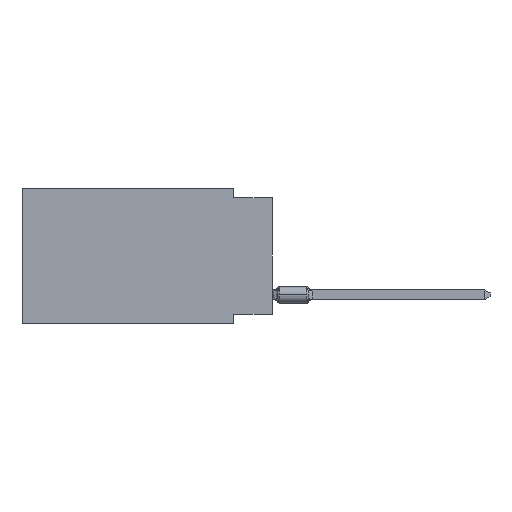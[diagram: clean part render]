
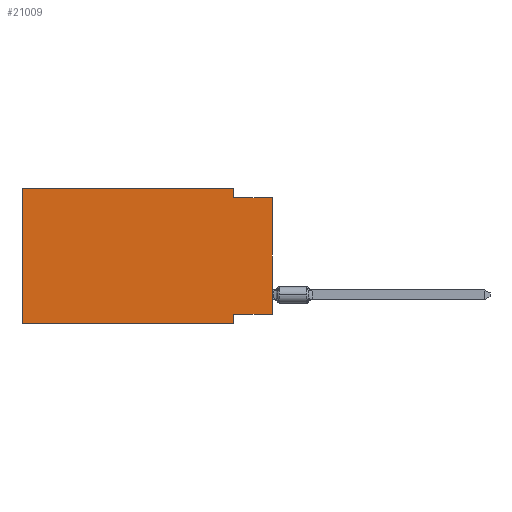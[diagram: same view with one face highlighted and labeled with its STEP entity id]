
A CAD part, left-side view. The second image highlights one B-rep face of the part: STEP entity #21009.
In plain terms, the highlighted planar face has unit normal (-1, 0, 0).
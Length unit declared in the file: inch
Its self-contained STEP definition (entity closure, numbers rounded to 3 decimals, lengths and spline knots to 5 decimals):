
#61 = CARTESIAN_POINT ( 'NONE',  ( 0., 0.645, 0. ) ) ;
#374 = EDGE_CURVE ( 'NONE', #6343, #25989, #20993, .T. ) ;
#680 = ORIENTED_EDGE ( 'NONE', *, *, #27275, .F. ) ;
#3112 = VECTOR ( 'NONE', #25550, 39.37008 ) ;
#3421 = DIRECTION ( 'NONE',  ( 1., 0., 0. ) ) ;
#3566 = CARTESIAN_POINT ( 'NONE',  ( 0., 0.645, 0. ) ) ;
#4497 = EDGE_CURVE ( 'NONE', #8063, #25989, #25173, .T. ) ;
#6343 = VERTEX_POINT ( 'NONE', #27596 ) ;
#6353 = VERTEX_POINT ( 'NONE', #24683 ) ;
#8007 = EDGE_CURVE ( 'NONE', #20018, #30855, #15881, .T. ) ;
#8063 = VERTEX_POINT ( 'NONE', #21209 ) ;
#8248 = VECTOR ( 'NONE', #24848, 39.37008 ) ;
#9344 = ORIENTED_EDGE ( 'NONE', *, *, #4497, .T. ) ;
#10070 = EDGE_CURVE ( 'NONE', #20807, #30855, #14075, .T. ) ;
#10418 = CARTESIAN_POINT ( 'NONE',  ( 0., 0.645, -0.35 ) ) ;
#10787 = AXIS2_PLACEMENT_3D ( 'NONE', #3566, #3421, #30625 ) ;
#10837 = ORIENTED_EDGE ( 'NONE', *, *, #8007, .T. ) ;
#11301 = DIRECTION ( 'NONE',  ( 0., -1., 0. ) ) ;
#12290 = CARTESIAN_POINT ( 'NONE',  ( 0., 0., -0.025 ) ) ;
#13291 = DIRECTION ( 'NONE',  ( 0., 0., 1. ) ) ;
#13655 = VECTOR ( 'NONE', #13291, 39.37008 ) ;
#14075 = LINE ( 'NONE', #19092, #23064 ) ;
#14401 = ORIENTED_EDGE ( 'NONE', *, *, #29085, .F. ) ;
#14994 = DIRECTION ( 'NONE',  ( 0., -1., 0. ) ) ;
#15822 = CARTESIAN_POINT ( 'NONE',  ( 0., 0.1, -0.35 ) ) ;
#15881 = LINE ( 'NONE', #20422, #13655 ) ;
#17553 = ORIENTED_EDGE ( 'NONE', *, *, #25008, .F. ) ;
#18621 = FACE_OUTER_BOUND ( 'NONE', #28024, .T. ) ;
#19092 = CARTESIAN_POINT ( 'NONE',  ( 0., 0., -0.025 ) ) ;
#19702 = DIRECTION ( 'NONE',  ( 0., 0., -1. ) ) ;
#19790 = CARTESIAN_POINT ( 'NONE',  ( 0., 0.1, -0.025 ) ) ;
#20018 = VERTEX_POINT ( 'NONE', #24718 ) ;
#20422 = CARTESIAN_POINT ( 'NONE',  ( 0., 0., 0. ) ) ;
#20581 = CARTESIAN_POINT ( 'NONE',  ( 0., 0.645, 0. ) ) ;
#20807 = VERTEX_POINT ( 'NONE', #19790 ) ;
#20993 = LINE ( 'NONE', #15822, #3112 ) ;
#21009 = ADVANCED_FACE ( 'NONE', ( #18621 ), #30462, .F. ) ;
#21209 = CARTESIAN_POINT ( 'NONE',  ( 0., 0.645, -0.35 ) ) ;
#21732 = CARTESIAN_POINT ( 'NONE',  ( 0., 0.1, -0.35 ) ) ;
#21948 = VECTOR ( 'NONE', #23014, 39.37008 ) ;
#22127 = CARTESIAN_POINT ( 'NONE',  ( 0., 0.645, 0. ) ) ;
#23014 = DIRECTION ( 'NONE',  ( 0., 0., 1. ) ) ;
#23064 = VECTOR ( 'NONE', #11301, 39.37008 ) ;
#24683 = CARTESIAN_POINT ( 'NONE',  ( 0., 0.1, 0. ) ) ;
#24718 = CARTESIAN_POINT ( 'NONE',  ( 0., 0., -0.325 ) ) ;
#24848 = DIRECTION ( 'NONE',  ( 0., -1., 0. ) ) ;
#24975 = EDGE_CURVE ( 'NONE', #6353, #20807, #31536, .T. ) ;
#25008 = EDGE_CURVE ( 'NONE', #25559, #6353, #31862, .T. ) ;
#25024 = VECTOR ( 'NONE', #14994, 39.37008 ) ;
#25173 = LINE ( 'NONE', #10418, #8248 ) ;
#25445 = ORIENTED_EDGE ( 'NONE', *, *, #10070, .F. ) ;
#25550 = DIRECTION ( 'NONE',  ( 0., 0., -1. ) ) ;
#25559 = VERTEX_POINT ( 'NONE', #61 ) ;
#25989 = VERTEX_POINT ( 'NONE', #21732 ) ;
#26591 = VECTOR ( 'NONE', #19702, 39.37008 ) ;
#26672 = ORIENTED_EDGE ( 'NONE', *, *, #374, .F. ) ;
#27275 = EDGE_CURVE ( 'NONE', #8063, #25559, #27742, .T. ) ;
#27596 = CARTESIAN_POINT ( 'NONE',  ( 0., 0.1, -0.325 ) ) ;
#27742 = LINE ( 'NONE', #20581, #21948 ) ;
#28024 = EDGE_LOOP ( 'NONE', ( #10837, #25445, #29255, #17553, #680, #9344, #26672, #14401 ) ) ;
#28168 = CARTESIAN_POINT ( 'NONE',  ( 0., 0., -0.325 ) ) ;
#28329 = LINE ( 'NONE', #28168, #31057 ) ;
#29085 = EDGE_CURVE ( 'NONE', #20018, #6343, #28329, .T. ) ;
#29255 = ORIENTED_EDGE ( 'NONE', *, *, #24975, .F. ) ;
#29426 = CARTESIAN_POINT ( 'NONE',  ( 0., 0.1, 0. ) ) ;
#30462 = PLANE ( 'NONE',  #10787 ) ;
#30625 = DIRECTION ( 'NONE',  ( 0., 0., -1. ) ) ;
#30855 = VERTEX_POINT ( 'NONE', #12290 ) ;
#31057 = VECTOR ( 'NONE', #31233, 39.37008 ) ;
#31233 = DIRECTION ( 'NONE',  ( 0., 1., 0. ) ) ;
#31536 = LINE ( 'NONE', #29426, #26591 ) ;
#31862 = LINE ( 'NONE', #22127, #25024 ) ;
